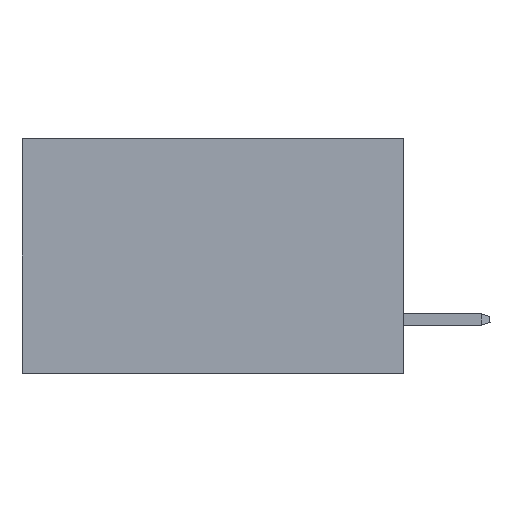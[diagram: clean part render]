
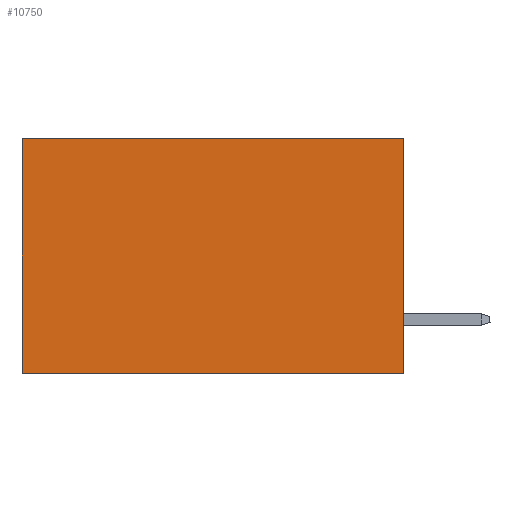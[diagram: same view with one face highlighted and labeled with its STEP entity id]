
A CAD part, left-side view. The second image highlights one B-rep face of the part: STEP entity #10750.
In plain terms, the highlighted planar face has unit normal (-1, 0, 0).
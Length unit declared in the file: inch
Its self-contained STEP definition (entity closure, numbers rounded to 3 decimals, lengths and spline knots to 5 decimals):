
#663 = FACE_OUTER_BOUND ( 'NONE', #9612, .T. ) ;
#1042 = CARTESIAN_POINT ( 'NONE',  ( 0.2875, 0., 0. ) ) ;
#1393 = VERTEX_POINT ( 'NONE', #26732 ) ;
#1602 = DIRECTION ( 'NONE',  ( 0., 0., -1. ) ) ;
#2000 = EDGE_CURVE ( 'NONE', #19647, #29956, #33429, .T. ) ;
#2975 = CARTESIAN_POINT ( 'NONE',  ( 0.2875, 0., 0. ) ) ;
#3592 = VECTOR ( 'NONE', #4487, 39.37008 ) ;
#3652 = LINE ( 'NONE', #20849, #21022 ) ;
#4487 = DIRECTION ( 'NONE',  ( 0., 0., -1. ) ) ;
#9284 = DIRECTION ( 'NONE',  ( 0., 0., -1. ) ) ;
#9612 = EDGE_LOOP ( 'NONE', ( #35282, #24324, #11957, #32875 ) ) ;
#10750 = ADVANCED_FACE ( 'NONE', ( #663 ), #34732, .F. ) ;
#11074 = VECTOR ( 'NONE', #1602, 39.37008 ) ;
#11528 = CARTESIAN_POINT ( 'NONE',  ( 0.2875, 0., -0.37 ) ) ;
#11957 = ORIENTED_EDGE ( 'NONE', *, *, #31772, .F. ) ;
#15830 = LINE ( 'NONE', #1042, #11074 ) ;
#16168 = DIRECTION ( 'NONE',  ( 0., 1., 0. ) ) ;
#16930 = CARTESIAN_POINT ( 'NONE',  ( 0.2875, 0.6, -0.37 ) ) ;
#19647 = VERTEX_POINT ( 'NONE', #11528 ) ;
#20501 = AXIS2_PLACEMENT_3D ( 'NONE', #26836, #26295, #9284 ) ;
#20849 = CARTESIAN_POINT ( 'NONE',  ( 0.2875, 0., 0. ) ) ;
#21022 = VECTOR ( 'NONE', #16168, 39.37008 ) ;
#22320 = VERTEX_POINT ( 'NONE', #2975 ) ;
#24324 = ORIENTED_EDGE ( 'NONE', *, *, #2000, .F. ) ;
#24625 = CARTESIAN_POINT ( 'NONE',  ( 0.2875, 0., -0.37 ) ) ;
#24841 = EDGE_CURVE ( 'NONE', #1393, #29956, #26931, .T. ) ;
#25182 = DIRECTION ( 'NONE',  ( 0., 1., 0. ) ) ;
#26295 = DIRECTION ( 'NONE',  ( 1., 0., 0. ) ) ;
#26732 = CARTESIAN_POINT ( 'NONE',  ( 0.2875, 0.6, 0. ) ) ;
#26751 = CARTESIAN_POINT ( 'NONE',  ( 0.2875, 0.6, 0. ) ) ;
#26836 = CARTESIAN_POINT ( 'NONE',  ( 0.2875, 0., 0. ) ) ;
#26931 = LINE ( 'NONE', #26751, #3592 ) ;
#28550 = EDGE_CURVE ( 'NONE', #22320, #1393, #3652, .T. ) ;
#29956 = VERTEX_POINT ( 'NONE', #16930 ) ;
#31772 = EDGE_CURVE ( 'NONE', #22320, #19647, #15830, .T. ) ;
#32875 = ORIENTED_EDGE ( 'NONE', *, *, #28550, .T. ) ;
#33429 = LINE ( 'NONE', #24625, #36484 ) ;
#34732 = PLANE ( 'NONE',  #20501 ) ;
#35282 = ORIENTED_EDGE ( 'NONE', *, *, #24841, .T. ) ;
#36484 = VECTOR ( 'NONE', #25182, 39.37008 ) ;
